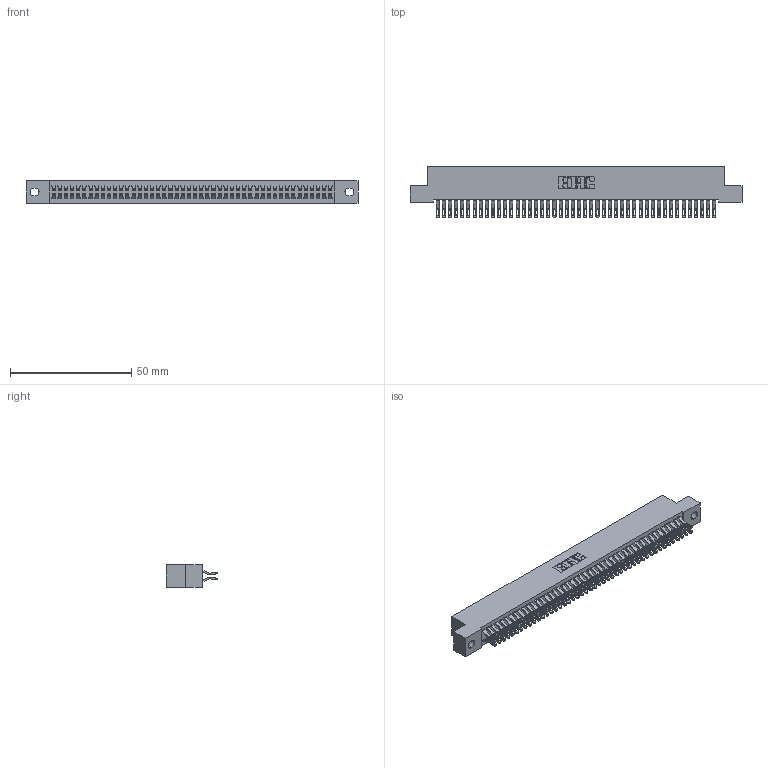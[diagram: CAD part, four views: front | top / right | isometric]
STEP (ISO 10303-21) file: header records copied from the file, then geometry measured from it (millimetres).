
FILE_DESCRIPTION (( 'STEP AP203' ), '1' );
FILE_NAME ('342-092-555-202.STEP', '2018-08-14T01:59:33', ( '' ), ( '' ), 'SwSTEP 2.0', 'SolidWorks 2016', '' );
FILE_SCHEMA (( 'CONFIG_CONTROL_DESIGN' ));
Length unit declared in the file: inch
Products named in the file (3): 342 Part_.128 Slot; 345-292-001_555 Tail; 342-092-555-202
Assembly tree (93 placements, depth 2):
  342-092-555-202
    342 Part_.128 Slot
    345-292-001_555 Tail  x92
Bounding box: 137.16 x 21.47 x 9.4 mm (x, y, z)
Volume: 12546.3 mm3; surface area: 21170.4 mm2
Topology: 93 solids, 93 shells, 5450 faces, 17147 edges, 11430 vertices
Faces by surface type: plane 3198, cylinder 2252
Entity records: 29405 total; most frequent: CARTESIAN_POINT 4904, ORIENTED_EDGE 4810, DIRECTION 4153, EDGE_CURVE 2405, VECTOR 2257, LINE 2257, VERTEX_POINT 1602, AXIS2_PLACEMENT_3D 948
